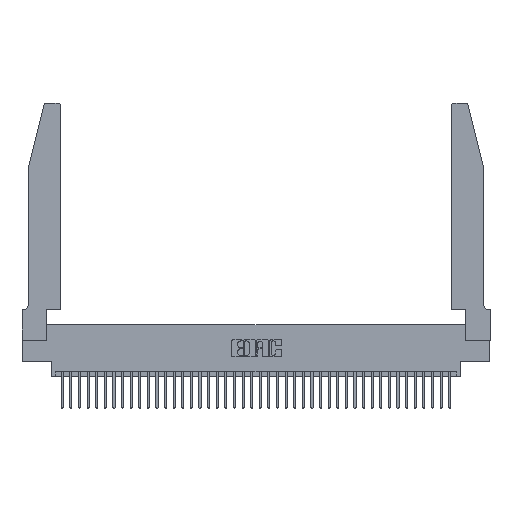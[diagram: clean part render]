
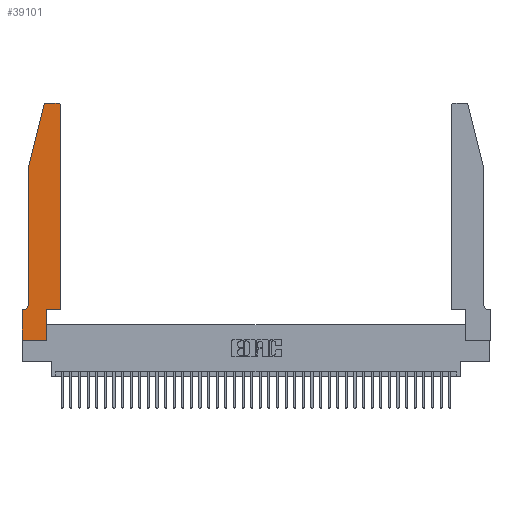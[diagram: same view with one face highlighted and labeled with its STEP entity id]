
A CAD part, top view. The second image highlights one B-rep face of the part: STEP entity #39101.
In plain terms, the highlighted planar face has unit normal (0, 0, 1).
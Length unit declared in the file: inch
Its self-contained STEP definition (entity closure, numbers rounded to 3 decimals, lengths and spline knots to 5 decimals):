
#167 = VERTEX_POINT ( 'NONE', #27376 ) ;
#689 = EDGE_CURVE ( 'NONE', #16209, #28843, #16909, .T. ) ;
#1039 = DIRECTION ( 'NONE',  ( 0., 0., -1. ) ) ;
#1163 = CARTESIAN_POINT ( 'NONE',  ( 0.0055, 0.42, 0.37 ) ) ;
#2237 = VECTOR ( 'NONE', #33125, 39.37008 ) ;
#2475 = CARTESIAN_POINT ( 'NONE',  ( 0.4505, 0.35, 0.37 ) ) ;
#2765 = LINE ( 'NONE', #39178, #2237 ) ;
#2817 = AXIS2_PLACEMENT_3D ( 'NONE', #21022, #12643, #18545 ) ;
#3236 = CARTESIAN_POINT ( 'NONE',  ( 0.284, 2.72, 0.37 ) ) ;
#3730 = DIRECTION ( 'NONE',  ( 0., 1., 0. ) ) ;
#4224 = PLANE ( 'NONE',  #28650 ) ;
#4239 = VERTEX_POINT ( 'NONE', #37650 ) ;
#6388 = EDGE_CURVE ( 'NONE', #17645, #29776, #29860, .T. ) ;
#6769 = ORIENTED_EDGE ( 'NONE', *, *, #21295, .T. ) ;
#7190 = CARTESIAN_POINT ( 'NONE',  ( 0., 0.35, 0.37 ) ) ;
#8589 = VERTEX_POINT ( 'NONE', #29492 ) ;
#9251 = EDGE_CURVE ( 'NONE', #31223, #18866, #12598, .T. ) ;
#10107 = ORIENTED_EDGE ( 'NONE', *, *, #37407, .T. ) ;
#10404 = AXIS2_PLACEMENT_3D ( 'NONE', #3236, #30983, #28141 ) ;
#11379 = FACE_OUTER_BOUND ( 'NONE', #32598, .T. ) ;
#11936 = VECTOR ( 'NONE', #35483, 39.37008 ) ;
#12598 = CIRCLE ( 'NONE', #15767, 0.07 ) ;
#12643 = DIRECTION ( 'NONE',  ( 0., 0., 1. ) ) ;
#12925 = LINE ( 'NONE', #20928, #34943 ) ;
#13476 = CARTESIAN_POINT ( 'NONE',  ( 0., 0., 0.37 ) ) ;
#13490 = VECTOR ( 'NONE', #25026, 39.37008 ) ;
#13673 = ORIENTED_EDGE ( 'NONE', *, *, #31950, .T. ) ;
#14407 = LINE ( 'NONE', #24729, #28561 ) ;
#15097 = VECTOR ( 'NONE', #3730, 39.37008 ) ;
#15131 = ORIENTED_EDGE ( 'NONE', *, *, #26689, .T. ) ;
#15135 = VECTOR ( 'NONE', #16632, 39.37008 ) ;
#15556 = ORIENTED_EDGE ( 'NONE', *, *, #689, .T. ) ;
#15767 = AXIS2_PLACEMENT_3D ( 'NONE', #1163, #1039, #29342 ) ;
#16209 = VERTEX_POINT ( 'NONE', #33186 ) ;
#16632 = DIRECTION ( 'NONE',  ( 1., 0., 0. ) ) ;
#16887 = CARTESIAN_POINT ( 'NONE',  ( 0.0755, 0.35, 0.37 ) ) ;
#16909 = LINE ( 'NONE', #2475, #13490 ) ;
#17645 = VERTEX_POINT ( 'NONE', #33647 ) ;
#18144 = LINE ( 'NONE', #31824, #33788 ) ;
#18545 = DIRECTION ( 'NONE',  ( 1., 0., 0. ) ) ;
#18866 = VERTEX_POINT ( 'NONE', #28027 ) ;
#19055 = ORIENTED_EDGE ( 'NONE', *, *, #29851, .T. ) ;
#19292 = ORIENTED_EDGE ( 'NONE', *, *, #6388, .T. ) ;
#19593 = LINE ( 'NONE', #25130, #27925 ) ;
#20245 = LINE ( 'NONE', #16887, #11936 ) ;
#20928 = CARTESIAN_POINT ( 'NONE',  ( 0.0755, 2., 0.37 ) ) ;
#21022 = CARTESIAN_POINT ( 'NONE',  ( 0.4205, 2.72, 0.37 ) ) ;
#21295 = EDGE_CURVE ( 'NONE', #8589, #31993, #12925, .T. ) ;
#22978 = CIRCLE ( 'NONE', #10404, 0.03 ) ;
#23095 = DIRECTION ( 'NONE',  ( 0., 0., 1. ) ) ;
#23915 = EDGE_CURVE ( 'NONE', #4239, #8589, #22978, .T. ) ;
#24010 = ORIENTED_EDGE ( 'NONE', *, *, #26372, .T. ) ;
#24729 = CARTESIAN_POINT ( 'NONE',  ( 0., 0., 0.37 ) ) ;
#24916 = CARTESIAN_POINT ( 'NONE',  ( 0.0755, 0.42, 0.37 ) ) ;
#25008 = DIRECTION ( 'NONE',  ( 0., -1., 0. ) ) ;
#25026 = DIRECTION ( 'NONE',  ( 1., 0., 0. ) ) ;
#25130 = CARTESIAN_POINT ( 'NONE',  ( 0.0755, 2., 0.37 ) ) ;
#25392 = LINE ( 'NONE', #13476, #15135 ) ;
#26372 = EDGE_CURVE ( 'NONE', #167, #35046, #25392, .T. ) ;
#26689 = EDGE_CURVE ( 'NONE', #28843, #17645, #36643, .T. ) ;
#27376 = CARTESIAN_POINT ( 'NONE',  ( 0., 0., 0.37 ) ) ;
#27694 = ORIENTED_EDGE ( 'NONE', *, *, #40342, .T. ) ;
#27925 = VECTOR ( 'NONE', #25008, 39.37008 ) ;
#28027 = CARTESIAN_POINT ( 'NONE',  ( 0.0055, 0.35, 0.37 ) ) ;
#28141 = DIRECTION ( 'NONE',  ( 1., 0., 0. ) ) ;
#28552 = DIRECTION ( 'NONE',  ( -1., 0., 0. ) ) ;
#28561 = VECTOR ( 'NONE', #40043, 39.37008 ) ;
#28650 = AXIS2_PLACEMENT_3D ( 'NONE', #7190, #23095, #35807 ) ;
#28843 = VERTEX_POINT ( 'NONE', #32661 ) ;
#29342 = DIRECTION ( 'NONE',  ( -1., 0., 0. ) ) ;
#29492 = CARTESIAN_POINT ( 'NONE',  ( 0.25487, 2.72718, 0.37 ) ) ;
#29776 = VERTEX_POINT ( 'NONE', #33841 ) ;
#29851 = EDGE_CURVE ( 'NONE', #18866, #36992, #20245, .T. ) ;
#29860 = CIRCLE ( 'NONE', #2817, 0.03 ) ;
#30592 = DIRECTION ( 'NONE',  ( -0.239, -0.971, 0. ) ) ;
#30909 = CARTESIAN_POINT ( 'NONE',  ( 0., 0.35, 0.37 ) ) ;
#30983 = DIRECTION ( 'NONE',  ( 0., 0., 1. ) ) ;
#31223 = VERTEX_POINT ( 'NONE', #24916 ) ;
#31645 = CARTESIAN_POINT ( 'NONE',  ( 0.2865, 0., 0.37 ) ) ;
#31824 = CARTESIAN_POINT ( 'NONE',  ( 0.2605, 2.75, 0.37 ) ) ;
#31950 = EDGE_CURVE ( 'NONE', #31993, #31223, #19593, .T. ) ;
#31993 = VERTEX_POINT ( 'NONE', #37202 ) ;
#32101 = EDGE_CURVE ( 'NONE', #29776, #4239, #18144, .T. ) ;
#32598 = EDGE_LOOP ( 'NONE', ( #34835, #37404, #6769, #13673, #35113, #19055, #10107, #24010, #27694, #15556, #15131, #19292 ) ) ;
#32661 = CARTESIAN_POINT ( 'NONE',  ( 0.4505, 0.35, 0.37 ) ) ;
#33125 = DIRECTION ( 'NONE',  ( 0., 1., 0. ) ) ;
#33186 = CARTESIAN_POINT ( 'NONE',  ( 0.2865, 0.35, 0.37 ) ) ;
#33647 = CARTESIAN_POINT ( 'NONE',  ( 0.4505, 2.72, 0.37 ) ) ;
#33788 = VECTOR ( 'NONE', #28552, 39.37008 ) ;
#33841 = CARTESIAN_POINT ( 'NONE',  ( 0.4205, 2.75, 0.37 ) ) ;
#34644 = CARTESIAN_POINT ( 'NONE',  ( 0.4505, 0.35, 0.37 ) ) ;
#34835 = ORIENTED_EDGE ( 'NONE', *, *, #32101, .T. ) ;
#34943 = VECTOR ( 'NONE', #30592, 39.37008 ) ;
#35046 = VERTEX_POINT ( 'NONE', #31645 ) ;
#35113 = ORIENTED_EDGE ( 'NONE', *, *, #9251, .T. ) ;
#35483 = DIRECTION ( 'NONE',  ( -1., 0., 0. ) ) ;
#35807 = DIRECTION ( 'NONE',  ( 1., 0., 0. ) ) ;
#36643 = LINE ( 'NONE', #34644, #15097 ) ;
#36992 = VERTEX_POINT ( 'NONE', #30909 ) ;
#37202 = CARTESIAN_POINT ( 'NONE',  ( 0.0755, 2., 0.37 ) ) ;
#37404 = ORIENTED_EDGE ( 'NONE', *, *, #23915, .T. ) ;
#37407 = EDGE_CURVE ( 'NONE', #36992, #167, #14407, .T. ) ;
#37650 = CARTESIAN_POINT ( 'NONE',  ( 0.284, 2.75, 0.37 ) ) ;
#39101 = ADVANCED_FACE ( 'NONE', ( #11379 ), #4224, .T. ) ;
#39178 = CARTESIAN_POINT ( 'NONE',  ( 0.2865, 0.35, 0.37 ) ) ;
#40043 = DIRECTION ( 'NONE',  ( 0., -1., 0. ) ) ;
#40342 = EDGE_CURVE ( 'NONE', #35046, #16209, #2765, .T. ) ;
